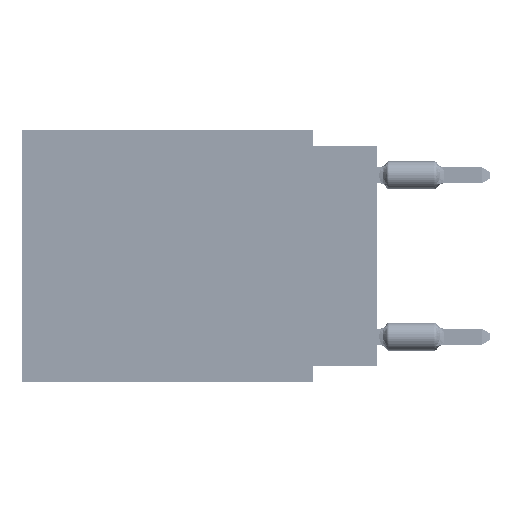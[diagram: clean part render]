
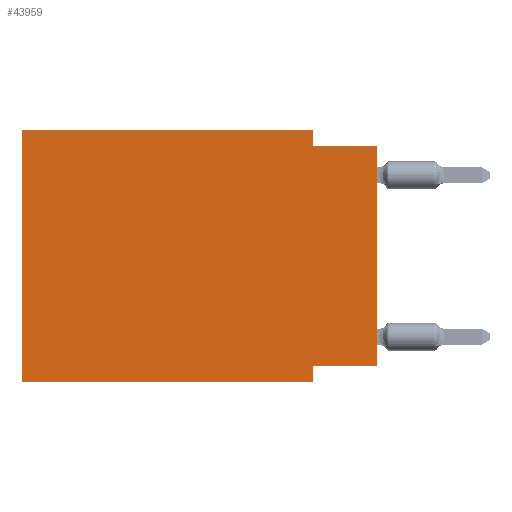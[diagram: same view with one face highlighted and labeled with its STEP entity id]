
A CAD part, left-side view. The second image highlights one B-rep face of the part: STEP entity #43959.
In plain terms, the highlighted planar face has unit normal (-1, 0, 0).
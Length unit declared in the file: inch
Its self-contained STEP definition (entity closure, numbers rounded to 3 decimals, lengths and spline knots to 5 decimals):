
#3124 = VERTEX_POINT ( 'NONE', #12217 ) ;
#3153 = ORIENTED_EDGE ( 'NONE', *, *, #7866, .F. ) ;
#4536 = DIRECTION ( 'NONE',  ( 0., 0., 1. ) ) ;
#4700 = ORIENTED_EDGE ( 'NONE', *, *, #63087, .T. ) ;
#5158 = ORIENTED_EDGE ( 'NONE', *, *, #8453, .F. ) ;
#5689 = LINE ( 'NONE', #70733, #9344 ) ;
#6762 = LINE ( 'NONE', #60821, #67148 ) ;
#6919 = EDGE_CURVE ( 'NONE', #22458, #68577, #22742, .T. ) ;
#7866 = EDGE_CURVE ( 'NONE', #62812, #11609, #5689, .T. ) ;
#8453 = EDGE_CURVE ( 'NONE', #68577, #43701, #6762, .T. ) ;
#8894 = EDGE_CURVE ( 'NONE', #3124, #55003, #28814, .T. ) ;
#9344 = VECTOR ( 'NONE', #76986, 39.37008 ) ;
#9448 = VERTEX_POINT ( 'NONE', #28346 ) ;
#9945 = ORIENTED_EDGE ( 'NONE', *, *, #51109, .F. ) ;
#11609 = VERTEX_POINT ( 'NONE', #16637 ) ;
#12217 = CARTESIAN_POINT ( 'NONE',  ( 0., 0.55, -0.39 ) ) ;
#13636 = LINE ( 'NONE', #57071, #29599 ) ;
#14449 = CARTESIAN_POINT ( 'NONE',  ( 0., 0.1, -0.025 ) ) ;
#16637 = CARTESIAN_POINT ( 'NONE',  ( 0., 0.1, -0.365 ) ) ;
#17021 = CARTESIAN_POINT ( 'NONE',  ( 0., 0., 0. ) ) ;
#17445 = CARTESIAN_POINT ( 'NONE',  ( 0., 0., -0.025 ) ) ;
#18273 = CARTESIAN_POINT ( 'NONE',  ( 0., 0., -0.365 ) ) ;
#20319 = CARTESIAN_POINT ( 'NONE',  ( 0., 0.1, -0.39 ) ) ;
#21294 = DIRECTION ( 'NONE',  ( 0., 0., -1. ) ) ;
#21939 = VECTOR ( 'NONE', #46633, 39.37008 ) ;
#22458 = VERTEX_POINT ( 'NONE', #50511 ) ;
#22742 = LINE ( 'NONE', #33700, #21939 ) ;
#28346 = CARTESIAN_POINT ( 'NONE',  ( 0., 0.1, -0.39 ) ) ;
#28814 = LINE ( 'NONE', #75075, #74702 ) ;
#29599 = VECTOR ( 'NONE', #37519, 39.37008 ) ;
#30187 = VECTOR ( 'NONE', #43831, 39.37008 ) ;
#32198 = EDGE_CURVE ( 'NONE', #3124, #9448, #13636, .T. ) ;
#33231 = DIRECTION ( 'NONE',  ( 0., -1., 0. ) ) ;
#33610 = DIRECTION ( 'NONE',  ( 0., -1., 0. ) ) ;
#33700 = CARTESIAN_POINT ( 'NONE',  ( 0., 0.1, 0. ) ) ;
#37519 = DIRECTION ( 'NONE',  ( 0., -1., 0. ) ) ;
#39579 = AXIS2_PLACEMENT_3D ( 'NONE', #51061, #75726, #21294 ) ;
#40130 = LINE ( 'NONE', #17021, #56136 ) ;
#43701 = VERTEX_POINT ( 'NONE', #17445 ) ;
#43831 = DIRECTION ( 'NONE',  ( 0., 0., -1. ) ) ;
#43959 = ADVANCED_FACE ( 'NONE', ( #58496 ), #45962, .F. ) ;
#44711 = EDGE_CURVE ( 'NONE', #55003, #22458, #74408, .T. ) ;
#45962 = PLANE ( 'NONE',  #39579 ) ;
#46633 = DIRECTION ( 'NONE',  ( 0., 0., -1. ) ) ;
#47997 = CARTESIAN_POINT ( 'NONE',  ( 0., 0.55, 0. ) ) ;
#48313 = VECTOR ( 'NONE', #33610, 39.37008 ) ;
#50511 = CARTESIAN_POINT ( 'NONE',  ( 0., 0.1, 0. ) ) ;
#51061 = CARTESIAN_POINT ( 'NONE',  ( 0., 0.55, 0. ) ) ;
#51109 = EDGE_CURVE ( 'NONE', #11609, #9448, #54812, .T. ) ;
#52233 = ORIENTED_EDGE ( 'NONE', *, *, #32198, .T. ) ;
#54046 = EDGE_LOOP ( 'NONE', ( #4700, #5158, #70824, #54440, #73597, #52233, #9945, #3153 ) ) ;
#54440 = ORIENTED_EDGE ( 'NONE', *, *, #44711, .F. ) ;
#54812 = LINE ( 'NONE', #20319, #30187 ) ;
#55003 = VERTEX_POINT ( 'NONE', #47997 ) ;
#56136 = VECTOR ( 'NONE', #75382, 39.37008 ) ;
#57071 = CARTESIAN_POINT ( 'NONE',  ( 0., 0.55, -0.39 ) ) ;
#58496 = FACE_OUTER_BOUND ( 'NONE', #54046, .T. ) ;
#60821 = CARTESIAN_POINT ( 'NONE',  ( 0., 0., -0.025 ) ) ;
#62812 = VERTEX_POINT ( 'NONE', #18273 ) ;
#63087 = EDGE_CURVE ( 'NONE', #62812, #43701, #40130, .T. ) ;
#67148 = VECTOR ( 'NONE', #33231, 39.37008 ) ;
#68577 = VERTEX_POINT ( 'NONE', #14449 ) ;
#68887 = CARTESIAN_POINT ( 'NONE',  ( 0., 0.55, 0. ) ) ;
#70733 = CARTESIAN_POINT ( 'NONE',  ( 0., 0., -0.365 ) ) ;
#70824 = ORIENTED_EDGE ( 'NONE', *, *, #6919, .F. ) ;
#73597 = ORIENTED_EDGE ( 'NONE', *, *, #8894, .F. ) ;
#74408 = LINE ( 'NONE', #68887, #48313 ) ;
#74702 = VECTOR ( 'NONE', #4536, 39.37008 ) ;
#75075 = CARTESIAN_POINT ( 'NONE',  ( 0., 0.55, 0. ) ) ;
#75382 = DIRECTION ( 'NONE',  ( 0., 0., 1. ) ) ;
#75726 = DIRECTION ( 'NONE',  ( 1., 0., 0. ) ) ;
#76986 = DIRECTION ( 'NONE',  ( 0., 1., 0. ) ) ;
